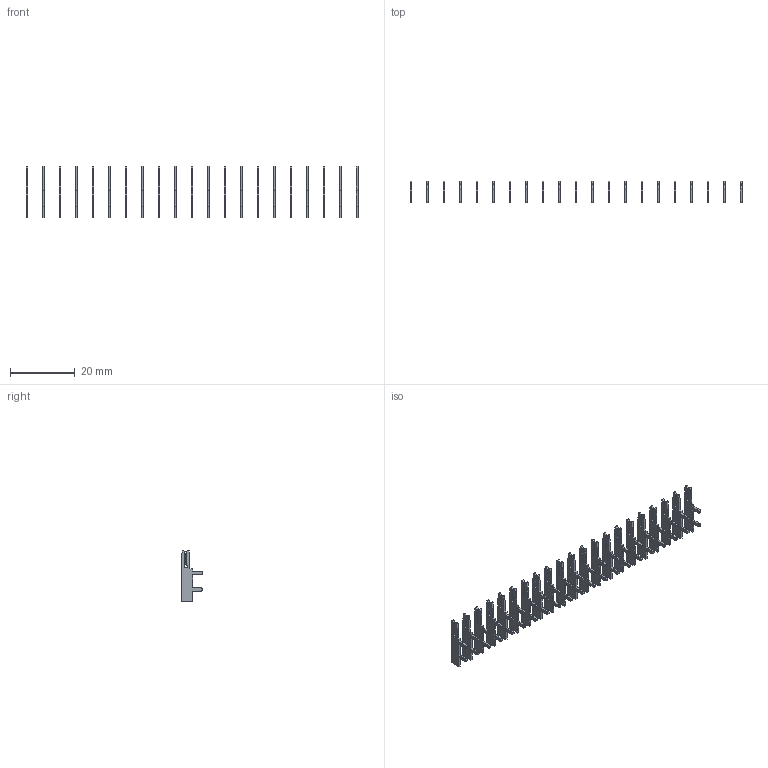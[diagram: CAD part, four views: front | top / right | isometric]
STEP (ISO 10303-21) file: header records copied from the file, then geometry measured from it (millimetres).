
FILE_DESCRIPTION (( 'STEP AP203' ), '1' );
FILE_NAME ('105-021-202-200.STEP', '2020-04-07T22:59:21', ( '' ), ( '' ), 'SwSTEP 2.0', 'SolidWorks 2016', '' );
FILE_SCHEMA (( 'CONFIG_CONTROL_DESIGN' ));
Length unit declared in the file: inch
Products named in the file (2): 100-290-001_100-290-202; 105-021-202-200
Assembly tree (21 placements, depth 2):
  105-021-202-200
    100-290-001_100-290-202  x21
Bounding box: 102.2 x 6.53 x 15.88 mm (x, y, z)
Volume: 667.2 mm3; surface area: 2967.3 mm2
Topology: 21 solids, 21 shells, 630 faces, 1764 edges, 1176 vertices
Faces by surface type: plane 483, cylinder 147
Entity records: 1802 total; most frequent: CARTESIAN_POINT 206, DIRECTION 202, ORIENTED_EDGE 168, EDGE_CURVE 84, AXIS2_PLACEMENT_3D 68, LINE 66, VECTOR 66, VERTEX_POINT 56
